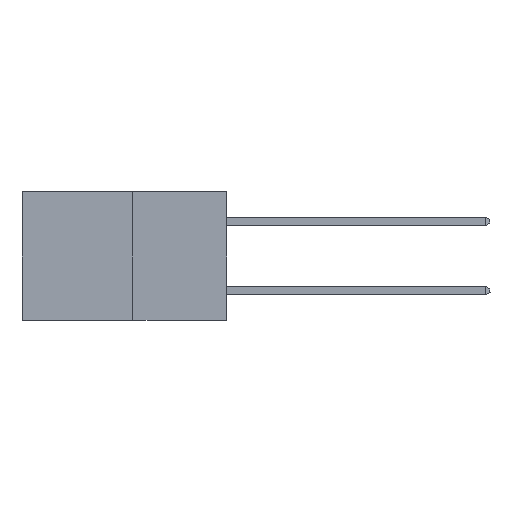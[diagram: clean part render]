
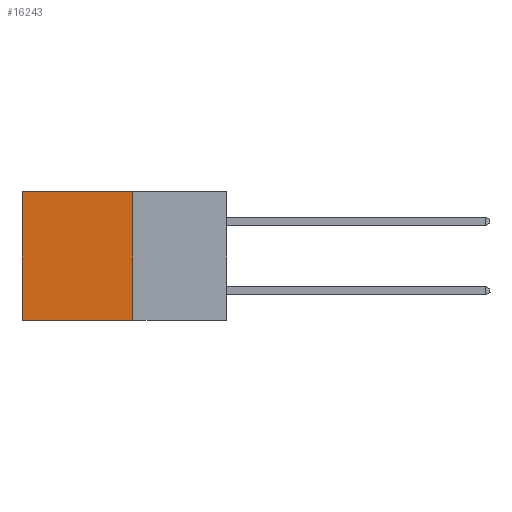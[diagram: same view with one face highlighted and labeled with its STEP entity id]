
A CAD part, left-side view. The second image highlights one B-rep face of the part: STEP entity #16243.
In plain terms, the highlighted planar face has unit normal (-1, 0, 0).
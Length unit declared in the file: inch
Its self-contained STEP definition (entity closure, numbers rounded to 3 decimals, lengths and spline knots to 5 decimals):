
#280 = VERTEX_POINT ( 'NONE', #15784 ) ;
#2241 = CARTESIAN_POINT ( 'NONE',  ( 0.277, 0.27, -0.37 ) ) ;
#2288 = VECTOR ( 'NONE', #9279, 39.37008 ) ;
#2387 = ORIENTED_EDGE ( 'NONE', *, *, #16790, .F. ) ;
#3245 = VECTOR ( 'NONE', #4754, 39.37008 ) ;
#3743 = EDGE_CURVE ( 'NONE', #28819, #280, #26811, .T. ) ;
#4754 = DIRECTION ( 'NONE',  ( 0., 0., -1. ) ) ;
#5331 = PLANE ( 'NONE',  #6979 ) ;
#6113 = ORIENTED_EDGE ( 'NONE', *, *, #19333, .T. ) ;
#6205 = DIRECTION ( 'NONE',  ( 0., 0., -1. ) ) ;
#6304 = CARTESIAN_POINT ( 'NONE',  ( 0.277, 0.59, -0.37 ) ) ;
#6939 = DIRECTION ( 'NONE',  ( 0., 1., 0. ) ) ;
#6979 = AXIS2_PLACEMENT_3D ( 'NONE', #22615, #12983, #29840 ) ;
#6997 = LINE ( 'NONE', #18480, #22315 ) ;
#7071 = ORIENTED_EDGE ( 'NONE', *, *, #3743, .T. ) ;
#9279 = DIRECTION ( 'NONE',  ( 0., 1., 0. ) ) ;
#10127 = LINE ( 'NONE', #24043, #23047 ) ;
#10377 = CARTESIAN_POINT ( 'NONE',  ( 0.277, 0.27, -0.37 ) ) ;
#11889 = ORIENTED_EDGE ( 'NONE', *, *, #23102, .F. ) ;
#12983 = DIRECTION ( 'NONE',  ( 1., 0., 0. ) ) ;
#15784 = CARTESIAN_POINT ( 'NONE',  ( 0.277, 0.59, 0. ) ) ;
#16243 = ADVANCED_FACE ( 'NONE', ( #24408 ), #5331, .F. ) ;
#16790 = EDGE_CURVE ( 'NONE', #28819, #17882, #17195, .T. ) ;
#17195 = LINE ( 'NONE', #2241, #3245 ) ;
#17882 = VERTEX_POINT ( 'NONE', #10377 ) ;
#18480 = CARTESIAN_POINT ( 'NONE',  ( 0.277, 0.59, -0.37 ) ) ;
#19333 = EDGE_CURVE ( 'NONE', #280, #19350, #6997, .T. ) ;
#19350 = VERTEX_POINT ( 'NONE', #6304 ) ;
#21826 = EDGE_LOOP ( 'NONE', ( #6113, #11889, #2387, #7071 ) ) ;
#22315 = VECTOR ( 'NONE', #6205, 39.37008 ) ;
#22615 = CARTESIAN_POINT ( 'NONE',  ( 0.277, 0.27, -0.37 ) ) ;
#23047 = VECTOR ( 'NONE', #6939, 39.37008 ) ;
#23102 = EDGE_CURVE ( 'NONE', #17882, #19350, #10127, .T. ) ;
#24043 = CARTESIAN_POINT ( 'NONE',  ( 0.277, 0.27, -0.37 ) ) ;
#24408 = FACE_OUTER_BOUND ( 'NONE', #21826, .T. ) ;
#26811 = LINE ( 'NONE', #28844, #2288 ) ;
#26896 = CARTESIAN_POINT ( 'NONE',  ( 0.277, 0.27, 0. ) ) ;
#28819 = VERTEX_POINT ( 'NONE', #26896 ) ;
#28844 = CARTESIAN_POINT ( 'NONE',  ( 0.277, 0.27, 0. ) ) ;
#29840 = DIRECTION ( 'NONE',  ( 0., 0., -1. ) ) ;
